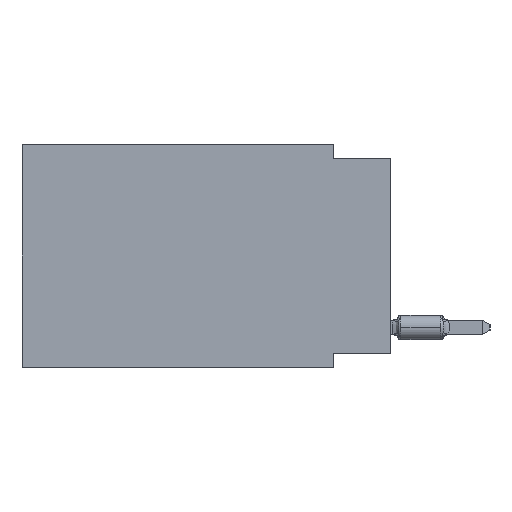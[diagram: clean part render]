
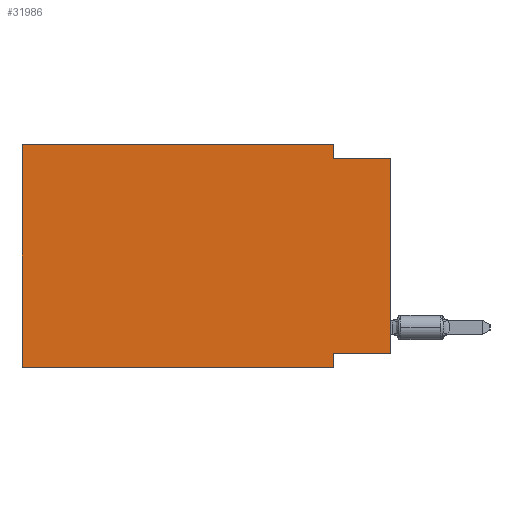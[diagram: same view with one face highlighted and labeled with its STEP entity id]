
A CAD part, left-side view. The second image highlights one B-rep face of the part: STEP entity #31986.
In plain terms, the highlighted planar face has unit normal (-1, 0, 0).
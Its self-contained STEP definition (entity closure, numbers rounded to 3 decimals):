
#932 = EDGE_CURVE ( 'NONE', #2255, #8596, #12770, .T. ) ;
#1190 = LINE ( 'NONE', #27897, #1871 ) ;
#1401 = CARTESIAN_POINT ( 'NONE',  ( 0., 0., 0. ) ) ;
#1409 = DIRECTION ( 'NONE',  ( 1., 0., 0. ) ) ;
#1871 = VECTOR ( 'NONE', #12578, 1000. ) ;
#2255 = VERTEX_POINT ( 'NONE', #10461 ) ;
#2620 = VERTEX_POINT ( 'NONE', #25417 ) ;
#3346 = LINE ( 'NONE', #18651, #25958 ) ;
#4358 = FACE_OUTER_BOUND ( 'NONE', #35669, .T. ) ;
#4585 = CARTESIAN_POINT ( 'NONE',  ( 0., 2.54, 0. ) ) ;
#5128 = CARTESIAN_POINT ( 'NONE',  ( 0., 16.383, 0. ) ) ;
#5435 = ORIENTED_EDGE ( 'NONE', *, *, #5698, .F. ) ;
#5442 = LINE ( 'NONE', #26429, #8230 ) ;
#5698 = EDGE_CURVE ( 'NONE', #10022, #21936, #15174, .T. ) ;
#5897 = CARTESIAN_POINT ( 'NONE',  ( 0., 2.54, 0. ) ) ;
#6301 = CARTESIAN_POINT ( 'NONE',  ( 0., 2.54, -9.271 ) ) ;
#7117 = DIRECTION ( 'NONE',  ( 0., 0., 1. ) ) ;
#7522 = LINE ( 'NONE', #4585, #35374 ) ;
#8230 = VECTOR ( 'NONE', #32711, 1000. ) ;
#8426 = AXIS2_PLACEMENT_3D ( 'NONE', #25553, #1409, #10456 ) ;
#8596 = VERTEX_POINT ( 'NONE', #13720 ) ;
#9103 = DIRECTION ( 'NONE',  ( 0., -1., 0. ) ) ;
#9402 = VECTOR ( 'NONE', #7117, 1000. ) ;
#9700 = CARTESIAN_POINT ( 'NONE',  ( 0., 16.383, 0. ) ) ;
#9934 = ORIENTED_EDGE ( 'NONE', *, *, #22413, .F. ) ;
#9985 = ORIENTED_EDGE ( 'NONE', *, *, #25542, .F. ) ;
#10022 = VERTEX_POINT ( 'NONE', #5128 ) ;
#10120 = ORIENTED_EDGE ( 'NONE', *, *, #11581, .F. ) ;
#10456 = DIRECTION ( 'NONE',  ( 0., 0., -1. ) ) ;
#10461 = CARTESIAN_POINT ( 'NONE',  ( 0., 2.54, -0.635 ) ) ;
#11581 = EDGE_CURVE ( 'NONE', #30058, #10022, #1190, .T. ) ;
#12578 = DIRECTION ( 'NONE',  ( 0., 0., 1. ) ) ;
#12770 = LINE ( 'NONE', #13344, #15140 ) ;
#12787 = ORIENTED_EDGE ( 'NONE', *, *, #31151, .T. ) ;
#12820 = LINE ( 'NONE', #1401, #9402 ) ;
#13344 = CARTESIAN_POINT ( 'NONE',  ( 0., 0., -0.635 ) ) ;
#13535 = VERTEX_POINT ( 'NONE', #6301 ) ;
#13720 = CARTESIAN_POINT ( 'NONE',  ( 0., 0., -0.635 ) ) ;
#15140 = VECTOR ( 'NONE', #19227, 1000. ) ;
#15174 = LINE ( 'NONE', #9700, #19178 ) ;
#16046 = ORIENTED_EDGE ( 'NONE', *, *, #19015, .F. ) ;
#16134 = DIRECTION ( 'NONE',  ( 0., -1., 0. ) ) ;
#18301 = CARTESIAN_POINT ( 'NONE',  ( 0., 0., -9.271 ) ) ;
#18651 = CARTESIAN_POINT ( 'NONE',  ( 0., 0., -9.271 ) ) ;
#19015 = EDGE_CURVE ( 'NONE', #35939, #13535, #3346, .T. ) ;
#19178 = VECTOR ( 'NONE', #9103, 1000. ) ;
#19227 = DIRECTION ( 'NONE',  ( 0., -1., 0. ) ) ;
#20353 = EDGE_CURVE ( 'NONE', #30058, #2620, #30845, .T. ) ;
#21334 = CARTESIAN_POINT ( 'NONE',  ( 0., 16.383, -9.906 ) ) ;
#21426 = CARTESIAN_POINT ( 'NONE',  ( 0., 16.383, -9.906 ) ) ;
#21936 = VERTEX_POINT ( 'NONE', #5897 ) ;
#22413 = EDGE_CURVE ( 'NONE', #21936, #2255, #7522, .T. ) ;
#24446 = ORIENTED_EDGE ( 'NONE', *, *, #20353, .T. ) ;
#25417 = CARTESIAN_POINT ( 'NONE',  ( 0., 2.54, -9.906 ) ) ;
#25542 = EDGE_CURVE ( 'NONE', #13535, #2620, #5442, .T. ) ;
#25553 = CARTESIAN_POINT ( 'NONE',  ( 0., 16.383, 0. ) ) ;
#25958 = VECTOR ( 'NONE', #27493, 1000. ) ;
#26148 = DIRECTION ( 'NONE',  ( 0., 0., -1. ) ) ;
#26429 = CARTESIAN_POINT ( 'NONE',  ( 0., 2.54, -9.906 ) ) ;
#27493 = DIRECTION ( 'NONE',  ( 0., 1., 0. ) ) ;
#27897 = CARTESIAN_POINT ( 'NONE',  ( 0., 16.383, 0. ) ) ;
#28079 = ORIENTED_EDGE ( 'NONE', *, *, #932, .F. ) ;
#28301 = PLANE ( 'NONE',  #8426 ) ;
#30058 = VERTEX_POINT ( 'NONE', #21334 ) ;
#30845 = LINE ( 'NONE', #21426, #32444 ) ;
#31151 = EDGE_CURVE ( 'NONE', #35939, #8596, #12820, .T. ) ;
#31986 = ADVANCED_FACE ( 'NONE', ( #4358 ), #28301, .F. ) ;
#32444 = VECTOR ( 'NONE', #16134, 1000. ) ;
#32711 = DIRECTION ( 'NONE',  ( 0., 0., -1. ) ) ;
#35374 = VECTOR ( 'NONE', #26148, 1000. ) ;
#35669 = EDGE_LOOP ( 'NONE', ( #12787, #28079, #9934, #5435, #10120, #24446, #9985, #16046 ) ) ;
#35939 = VERTEX_POINT ( 'NONE', #18301 ) ;
